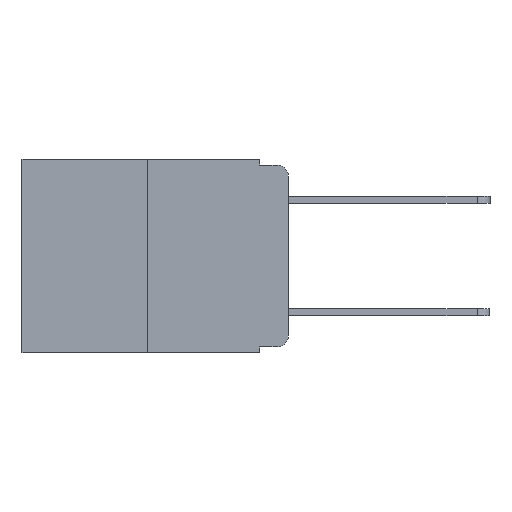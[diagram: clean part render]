
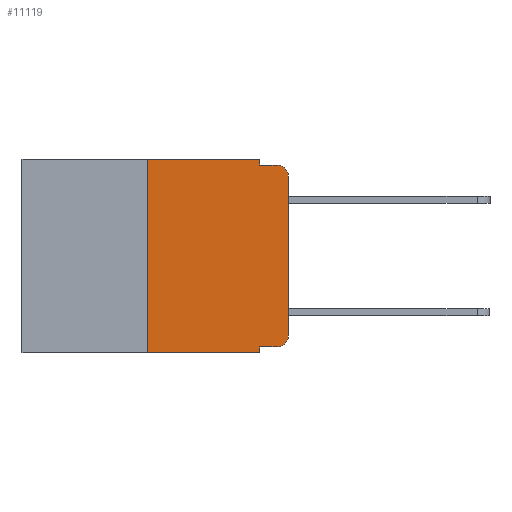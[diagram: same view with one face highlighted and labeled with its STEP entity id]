
A CAD part, left-side view. The second image highlights one B-rep face of the part: STEP entity #11119.
In plain terms, the highlighted planar face has unit normal (-1, 0, 0).
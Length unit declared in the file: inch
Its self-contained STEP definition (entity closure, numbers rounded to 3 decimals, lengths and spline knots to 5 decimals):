
#78 = CARTESIAN_POINT ( 'NONE',  ( 0., 0.25, 0. ) ) ;
#115 = ORIENTED_EDGE ( 'NONE', *, *, #4267, .T. ) ;
#136 = VERTEX_POINT ( 'NONE', #284 ) ;
#272 = VERTEX_POINT ( 'NONE', #5080 ) ;
#284 = CARTESIAN_POINT ( 'NONE',  ( 0., 0., -0.03 ) ) ;
#290 = ORIENTED_EDGE ( 'NONE', *, *, #2912, .T. ) ;
#305 = LINE ( 'NONE', #9860, #6842 ) ;
#312 = CARTESIAN_POINT ( 'NONE',  ( 0., 0.051, -0.01 ) ) ;
#442 = DIRECTION ( 'NONE',  ( 0., -1., 0. ) ) ;
#558 = AXIS2_PLACEMENT_3D ( 'NONE', #4294, #5059, #8579 ) ;
#688 = VERTEX_POINT ( 'NONE', #5212 ) ;
#837 = VECTOR ( 'NONE', #4947, 39.37008 ) ;
#839 = CARTESIAN_POINT ( 'NONE',  ( 0., 0.051, -0.343 ) ) ;
#865 = ORIENTED_EDGE ( 'NONE', *, *, #3443, .T. ) ;
#971 = CARTESIAN_POINT ( 'NONE',  ( 0., 0.051, -0.01 ) ) ;
#1180 = CARTESIAN_POINT ( 'NONE',  ( 0., 0.473, 0. ) ) ;
#1288 = VECTOR ( 'NONE', #1834, 39.37008 ) ;
#1415 = EDGE_CURVE ( 'NONE', #2398, #136, #6651, .T. ) ;
#1608 = PLANE ( 'NONE',  #3085 ) ;
#1639 = EDGE_CURVE ( 'NONE', #7746, #7259, #11004, .T. ) ;
#1737 = ORIENTED_EDGE ( 'NONE', *, *, #5718, .F. ) ;
#1807 = AXIS2_PLACEMENT_3D ( 'NONE', #9162, #9050, #8803 ) ;
#1834 = DIRECTION ( 'NONE',  ( 0., -1., 0. ) ) ;
#1885 = VECTOR ( 'NONE', #5292, 39.37008 ) ;
#1888 = ORIENTED_EDGE ( 'NONE', *, *, #5584, .F. ) ;
#2106 = CARTESIAN_POINT ( 'NONE',  ( 0., 0.051, -0.333 ) ) ;
#2398 = VERTEX_POINT ( 'NONE', #7140 ) ;
#2545 = VERTEX_POINT ( 'NONE', #8629 ) ;
#2813 = CIRCLE ( 'NONE', #558, 0.02 ) ;
#2912 = EDGE_CURVE ( 'NONE', #136, #688, #2813, .T. ) ;
#3085 = AXIS2_PLACEMENT_3D ( 'NONE', #4317, #10399, #5234 ) ;
#3147 = CARTESIAN_POINT ( 'NONE',  ( 0., 0., 0. ) ) ;
#3161 = LINE ( 'NONE', #2106, #837 ) ;
#3443 = EDGE_CURVE ( 'NONE', #272, #7259, #305, .T. ) ;
#3616 = DIRECTION ( 'NONE',  ( 0., 0., -1. ) ) ;
#3815 = CARTESIAN_POINT ( 'NONE',  ( 0., 0.051, -0.333 ) ) ;
#3875 = ORIENTED_EDGE ( 'NONE', *, *, #1639, .F. ) ;
#4116 = ORIENTED_EDGE ( 'NONE', *, *, #1415, .T. ) ;
#4267 = EDGE_CURVE ( 'NONE', #2545, #2398, #4705, .T. ) ;
#4294 = CARTESIAN_POINT ( 'NONE',  ( 0., 0.02, -0.03 ) ) ;
#4317 = CARTESIAN_POINT ( 'NONE',  ( 0., 0.473, 0. ) ) ;
#4387 = LINE ( 'NONE', #78, #11007 ) ;
#4616 = EDGE_CURVE ( 'NONE', #7746, #2545, #3161, .T. ) ;
#4705 = CIRCLE ( 'NONE', #1807, 0.02 ) ;
#4947 = DIRECTION ( 'NONE',  ( 0., -1., 0. ) ) ;
#5059 = DIRECTION ( 'NONE',  ( -1., 0., 0. ) ) ;
#5080 = CARTESIAN_POINT ( 'NONE',  ( 0., 0.25, -0.343 ) ) ;
#5212 = CARTESIAN_POINT ( 'NONE',  ( 0., 0.02, -0.01 ) ) ;
#5234 = DIRECTION ( 'NONE',  ( 0., 0., -1. ) ) ;
#5292 = DIRECTION ( 'NONE',  ( 0., 0., 1. ) ) ;
#5321 = VERTEX_POINT ( 'NONE', #6818 ) ;
#5584 = EDGE_CURVE ( 'NONE', #272, #5321, #4387, .T. ) ;
#5718 = EDGE_CURVE ( 'NONE', #5321, #6978, #7581, .T. ) ;
#6469 = CARTESIAN_POINT ( 'NONE',  ( 0., 0.051, 0. ) ) ;
#6488 = DIRECTION ( 'NONE',  ( 0., -1., 0. ) ) ;
#6651 = LINE ( 'NONE', #3147, #1885 ) ;
#6818 = CARTESIAN_POINT ( 'NONE',  ( 0., 0.25, 0. ) ) ;
#6842 = VECTOR ( 'NONE', #442, 39.37008 ) ;
#6978 = VERTEX_POINT ( 'NONE', #7511 ) ;
#7140 = CARTESIAN_POINT ( 'NONE',  ( 0., 0., -0.313 ) ) ;
#7259 = VERTEX_POINT ( 'NONE', #839 ) ;
#7322 = VECTOR ( 'NONE', #6488, 39.37008 ) ;
#7486 = DIRECTION ( 'NONE',  ( 0., 0., -1. ) ) ;
#7511 = CARTESIAN_POINT ( 'NONE',  ( 0., 0.051, 0. ) ) ;
#7581 = LINE ( 'NONE', #1180, #7322 ) ;
#7746 = VERTEX_POINT ( 'NONE', #3815 ) ;
#7997 = ORIENTED_EDGE ( 'NONE', *, *, #4616, .T. ) ;
#8030 = LINE ( 'NONE', #971, #1288 ) ;
#8579 = DIRECTION ( 'NONE',  ( 0., 0., -1. ) ) ;
#8629 = CARTESIAN_POINT ( 'NONE',  ( 0., 0.02, -0.333 ) ) ;
#8803 = DIRECTION ( 'NONE',  ( 0., 0., -1. ) ) ;
#8855 = CARTESIAN_POINT ( 'NONE',  ( 0., 0.051, 0. ) ) ;
#8941 = ORIENTED_EDGE ( 'NONE', *, *, #11243, .F. ) ;
#9050 = DIRECTION ( 'NONE',  ( -1., 0., 0. ) ) ;
#9162 = CARTESIAN_POINT ( 'NONE',  ( 0., 0.02, -0.313 ) ) ;
#9593 = VECTOR ( 'NONE', #7486, 39.37008 ) ;
#9804 = VECTOR ( 'NONE', #3616, 39.37008 ) ;
#9860 = CARTESIAN_POINT ( 'NONE',  ( 0., 0.473, -0.343 ) ) ;
#10065 = LINE ( 'NONE', #8855, #9804 ) ;
#10084 = EDGE_LOOP ( 'NONE', ( #4116, #290, #10671, #8941, #1737, #1888, #865, #3875, #7997, #115 ) ) ;
#10399 = DIRECTION ( 'NONE',  ( 1., 0., 0. ) ) ;
#10562 = DIRECTION ( 'NONE',  ( 0., 0., 1. ) ) ;
#10671 = ORIENTED_EDGE ( 'NONE', *, *, #11220, .F. ) ;
#10829 = FACE_OUTER_BOUND ( 'NONE', #10084, .T. ) ;
#10901 = VERTEX_POINT ( 'NONE', #312 ) ;
#11004 = LINE ( 'NONE', #6469, #9593 ) ;
#11007 = VECTOR ( 'NONE', #10562, 39.37008 ) ;
#11119 = ADVANCED_FACE ( 'NONE', ( #10829 ), #1608, .F. ) ;
#11220 = EDGE_CURVE ( 'NONE', #10901, #688, #8030, .T. ) ;
#11243 = EDGE_CURVE ( 'NONE', #6978, #10901, #10065, .T. ) ;
